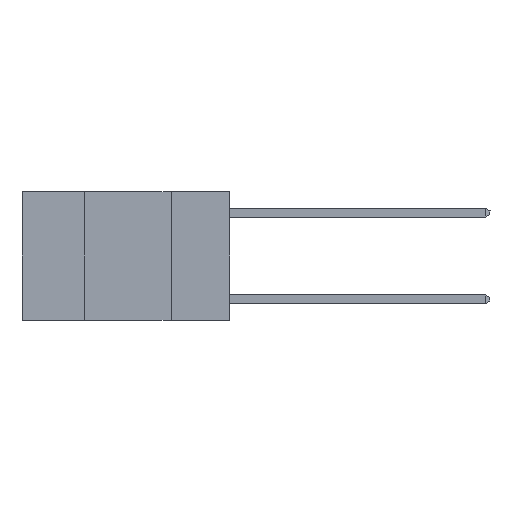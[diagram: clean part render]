
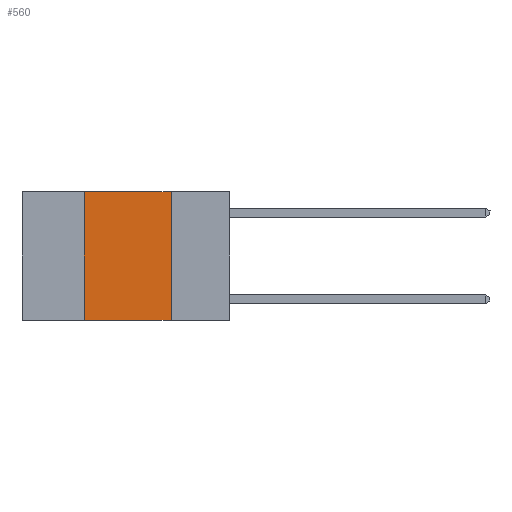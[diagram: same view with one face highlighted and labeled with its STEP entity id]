
A CAD part, left-side view. The second image highlights one B-rep face of the part: STEP entity #560.
In plain terms, the highlighted planar face has unit normal (-1, 0, 0).
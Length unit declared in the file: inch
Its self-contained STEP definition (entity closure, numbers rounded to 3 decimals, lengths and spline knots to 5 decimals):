
#356 = EDGE_CURVE ( 'NONE', #13423, #4579, #6269, .T. ) ;
#560 = ADVANCED_FACE ( 'NONE', ( #2839 ), #11025, .F. ) ;
#1028 = DIRECTION ( 'NONE',  ( 0., -1., 0. ) ) ;
#1589 = CARTESIAN_POINT ( 'NONE',  ( 0., 0.6, -0.37 ) ) ;
#1655 = CARTESIAN_POINT ( 'NONE',  ( 0., 0.42, 0. ) ) ;
#1927 = CARTESIAN_POINT ( 'NONE',  ( 0., 0.17, 0. ) ) ;
#2420 = CARTESIAN_POINT ( 'NONE',  ( 0., 0.17, 0. ) ) ;
#2839 = FACE_OUTER_BOUND ( 'NONE', #14027, .T. ) ;
#2870 = DIRECTION ( 'NONE',  ( 0., -1., 0. ) ) ;
#4115 = ORIENTED_EDGE ( 'NONE', *, *, #13983, .T. ) ;
#4579 = VERTEX_POINT ( 'NONE', #1927 ) ;
#4647 = VECTOR ( 'NONE', #2870, 39.37008 ) ;
#5067 = LINE ( 'NONE', #1589, #4647 ) ;
#5087 = LINE ( 'NONE', #12787, #8243 ) ;
#5729 = DIRECTION ( 'NONE',  ( 0., 0., -1. ) ) ;
#6083 = VERTEX_POINT ( 'NONE', #15572 ) ;
#6269 = LINE ( 'NONE', #6663, #13351 ) ;
#6663 = CARTESIAN_POINT ( 'NONE',  ( 0., 0.6, 0. ) ) ;
#8243 = VECTOR ( 'NONE', #15485, 39.37008 ) ;
#8705 = ORIENTED_EDGE ( 'NONE', *, *, #13726, .F. ) ;
#9287 = VECTOR ( 'NONE', #10522, 39.37008 ) ;
#10522 = DIRECTION ( 'NONE',  ( 0., 0., -1. ) ) ;
#11025 = PLANE ( 'NONE',  #13141 ) ;
#11995 = VERTEX_POINT ( 'NONE', #15396 ) ;
#12397 = LINE ( 'NONE', #2420, #9287 ) ;
#12787 = CARTESIAN_POINT ( 'NONE',  ( 0., 0.42, 0. ) ) ;
#13141 = AXIS2_PLACEMENT_3D ( 'NONE', #16299, #13701, #5729 ) ;
#13351 = VECTOR ( 'NONE', #1028, 39.37008 ) ;
#13423 = VERTEX_POINT ( 'NONE', #1655 ) ;
#13525 = EDGE_CURVE ( 'NONE', #6083, #13423, #5087, .T. ) ;
#13701 = DIRECTION ( 'NONE',  ( 1., 0., 0. ) ) ;
#13726 = EDGE_CURVE ( 'NONE', #4579, #11995, #12397, .T. ) ;
#13983 = EDGE_CURVE ( 'NONE', #6083, #11995, #5067, .T. ) ;
#14027 = EDGE_LOOP ( 'NONE', ( #8705, #14306, #15175, #4115 ) ) ;
#14306 = ORIENTED_EDGE ( 'NONE', *, *, #356, .F. ) ;
#15175 = ORIENTED_EDGE ( 'NONE', *, *, #13525, .F. ) ;
#15396 = CARTESIAN_POINT ( 'NONE',  ( 0., 0.17, -0.37 ) ) ;
#15485 = DIRECTION ( 'NONE',  ( 0., 0., 1. ) ) ;
#15572 = CARTESIAN_POINT ( 'NONE',  ( 0., 0.42, -0.37 ) ) ;
#16299 = CARTESIAN_POINT ( 'NONE',  ( 0., 0.6, 0. ) ) ;
